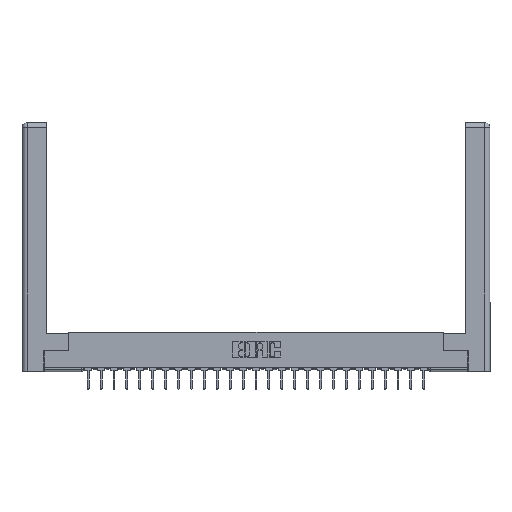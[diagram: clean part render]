
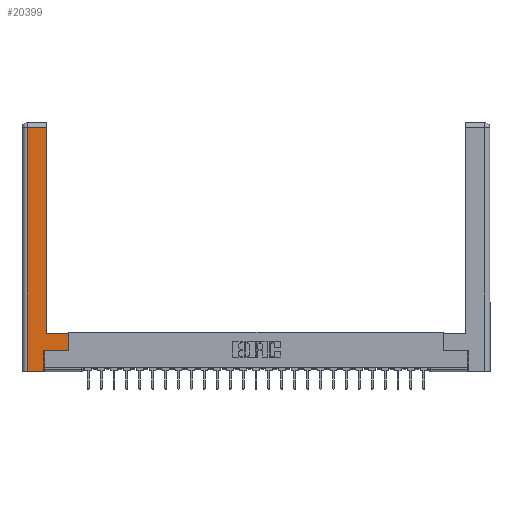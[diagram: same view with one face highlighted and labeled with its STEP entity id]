
A CAD part, top view. The second image highlights one B-rep face of the part: STEP entity #20399.
In plain terms, the highlighted planar face has unit normal (0, 0, 1).
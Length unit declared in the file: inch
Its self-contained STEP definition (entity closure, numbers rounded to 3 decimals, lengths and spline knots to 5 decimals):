
#208 = EDGE_CURVE ( 'NONE', #15063, #18840, #10611, .T. ) ;
#464 = CARTESIAN_POINT ( 'NONE',  ( 0.295, 3., 0. ) ) ;
#992 = ORIENTED_EDGE ( 'NONE', *, *, #26463, .T. ) ;
#1173 = CARTESIAN_POINT ( 'NONE',  ( 0.0615, 2.94, 0. ) ) ;
#1514 = DIRECTION ( 'NONE',  ( 1., 0., 0. ) ) ;
#1814 = CARTESIAN_POINT ( 'NONE',  ( 0.295, 2.94, 0. ) ) ;
#1885 = EDGE_LOOP ( 'NONE', ( #2380, #9185, #12257, #11818, #21707, #17428, #992, #10836 ) ) ;
#2359 = CARTESIAN_POINT ( 'NONE',  ( 0.265, 0.245, 0. ) ) ;
#2380 = ORIENTED_EDGE ( 'NONE', *, *, #14284, .T. ) ;
#2795 = VECTOR ( 'NONE', #10951, 39.37008 ) ;
#3325 = CARTESIAN_POINT ( 'NONE',  ( 0.565, 0.245, 0. ) ) ;
#5106 = LINE ( 'NONE', #16551, #20501 ) ;
#5296 = DIRECTION ( 'NONE',  ( -1., 0., 0. ) ) ;
#5474 = EDGE_CURVE ( 'NONE', #26819, #6677, #5991, .T. ) ;
#5991 = LINE ( 'NONE', #14200, #25304 ) ;
#6176 = VECTOR ( 'NONE', #23858, 39.37008 ) ;
#6377 = DIRECTION ( 'NONE',  ( 0., 1., 0. ) ) ;
#6677 = VERTEX_POINT ( 'NONE', #11639 ) ;
#6750 = VECTOR ( 'NONE', #1514, 39.37008 ) ;
#7492 = VECTOR ( 'NONE', #6377, 39.37008 ) ;
#7914 = DIRECTION ( 'NONE',  ( 0., -1., 0. ) ) ;
#9185 = ORIENTED_EDGE ( 'NONE', *, *, #21058, .T. ) ;
#9376 = DIRECTION ( 'NONE',  ( 0., 0., -1. ) ) ;
#9438 = LINE ( 'NONE', #12149, #6750 ) ;
#9566 = EDGE_CURVE ( 'NONE', #18074, #15063, #20906, .T. ) ;
#10611 = LINE ( 'NONE', #3325, #23619 ) ;
#10836 = ORIENTED_EDGE ( 'NONE', *, *, #21947, .T. ) ;
#10888 = EDGE_CURVE ( 'NONE', #6677, #18074, #9438, .T. ) ;
#10951 = DIRECTION ( 'NONE',  ( -1., 0., 0. ) ) ;
#11639 = CARTESIAN_POINT ( 'NONE',  ( 0.0615, 0., 0. ) ) ;
#11818 = ORIENTED_EDGE ( 'NONE', *, *, #10888, .T. ) ;
#12149 = CARTESIAN_POINT ( 'NONE',  ( 0.265, 0., 0. ) ) ;
#12257 = ORIENTED_EDGE ( 'NONE', *, *, #5474, .T. ) ;
#12366 = CARTESIAN_POINT ( 'NONE',  ( 0.295, 0.45, 0. ) ) ;
#12493 = VECTOR ( 'NONE', #5296, 39.37008 ) ;
#13602 = DIRECTION ( 'NONE',  ( -1., 0., 0. ) ) ;
#13814 = VERTEX_POINT ( 'NONE', #26723 ) ;
#14200 = CARTESIAN_POINT ( 'NONE',  ( 0.0615, 0., 0. ) ) ;
#14284 = EDGE_CURVE ( 'NONE', #25358, #23895, #16563, .T. ) ;
#15063 = VERTEX_POINT ( 'NONE', #22546 ) ;
#15736 = CARTESIAN_POINT ( 'NONE',  ( 0., 0., 0. ) ) ;
#16551 = CARTESIAN_POINT ( 'NONE',  ( 0.565, 0.45, 0. ) ) ;
#16563 = LINE ( 'NONE', #464, #6176 ) ;
#16937 = CARTESIAN_POINT ( 'NONE',  ( 0.265, 0., 0. ) ) ;
#17061 = AXIS2_PLACEMENT_3D ( 'NONE', #15736, #9376, #13602 ) ;
#17428 = ORIENTED_EDGE ( 'NONE', *, *, #208, .T. ) ;
#18074 = VERTEX_POINT ( 'NONE', #16937 ) ;
#18219 = DIRECTION ( 'NONE',  ( 1., 0., 0. ) ) ;
#18840 = VERTEX_POINT ( 'NONE', #25683 ) ;
#19544 = LINE ( 'NONE', #1173, #12493 ) ;
#20399 = ADVANCED_FACE ( 'NONE', ( #24835 ), #21896, .F. ) ;
#20501 = VECTOR ( 'NONE', #24963, 39.37008 ) ;
#20852 = LINE ( 'NONE', #23883, #2795 ) ;
#20906 = LINE ( 'NONE', #2359, #7492 ) ;
#21058 = EDGE_CURVE ( 'NONE', #23895, #26819, #19544, .T. ) ;
#21707 = ORIENTED_EDGE ( 'NONE', *, *, #9566, .T. ) ;
#21896 = PLANE ( 'NONE',  #17061 ) ;
#21947 = EDGE_CURVE ( 'NONE', #13814, #25358, #20852, .T. ) ;
#21999 = CARTESIAN_POINT ( 'NONE',  ( 0.0615, 2.94, 0. ) ) ;
#22546 = CARTESIAN_POINT ( 'NONE',  ( 0.265, 0.245, 0. ) ) ;
#23619 = VECTOR ( 'NONE', #18219, 39.37008 ) ;
#23858 = DIRECTION ( 'NONE',  ( 0., 1., 0. ) ) ;
#23883 = CARTESIAN_POINT ( 'NONE',  ( 0.295, 0.45, 0. ) ) ;
#23895 = VERTEX_POINT ( 'NONE', #1814 ) ;
#24835 = FACE_OUTER_BOUND ( 'NONE', #1885, .T. ) ;
#24963 = DIRECTION ( 'NONE',  ( 0., 1., 0. ) ) ;
#25304 = VECTOR ( 'NONE', #7914, 39.37008 ) ;
#25358 = VERTEX_POINT ( 'NONE', #12366 ) ;
#25683 = CARTESIAN_POINT ( 'NONE',  ( 0.565, 0.245, 0. ) ) ;
#26463 = EDGE_CURVE ( 'NONE', #18840, #13814, #5106, .T. ) ;
#26723 = CARTESIAN_POINT ( 'NONE',  ( 0.565, 0.45, 0. ) ) ;
#26819 = VERTEX_POINT ( 'NONE', #21999 ) ;
